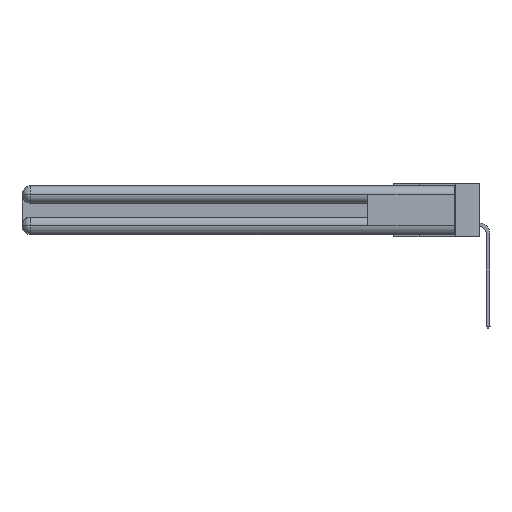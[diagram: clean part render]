
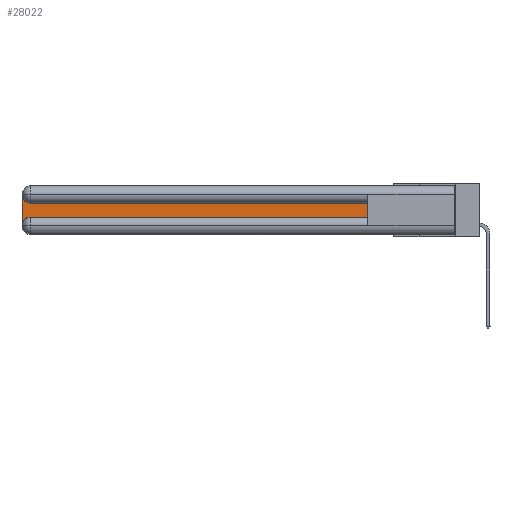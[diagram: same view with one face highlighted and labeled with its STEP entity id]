
A CAD part, left-side view. The second image highlights one B-rep face of the part: STEP entity #28022.
In plain terms, the highlighted planar face has unit normal (-1, 0, 0).
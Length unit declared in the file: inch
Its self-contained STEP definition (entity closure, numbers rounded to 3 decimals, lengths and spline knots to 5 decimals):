
#362 = CIRCLE ( 'NONE', #23428, 0.06 ) ;
#473 = ORIENTED_EDGE ( 'NONE', *, *, #30246, .T. ) ;
#719 = LINE ( 'NONE', #30095, #20214 ) ;
#2472 = ORIENTED_EDGE ( 'NONE', *, *, #22421, .T. ) ;
#3016 = CARTESIAN_POINT ( 'NONE',  ( 0.075, 2.94, -0.0625 ) ) ;
#3349 = VECTOR ( 'NONE', #31787, 39.37008 ) ;
#3365 = VERTEX_POINT ( 'NONE', #17235 ) ;
#3503 = PLANE ( 'NONE',  #10403 ) ;
#5571 = CIRCLE ( 'NONE', #5984, 0.06 ) ;
#5984 = AXIS2_PLACEMENT_3D ( 'NONE', #3016, #10112, #27837 ) ;
#6042 = VERTEX_POINT ( 'NONE', #25935 ) ;
#6546 = ORIENTED_EDGE ( 'NONE', *, *, #10411, .T. ) ;
#7723 = VERTEX_POINT ( 'NONE', #15657 ) ;
#8733 = DIRECTION ( 'NONE',  ( 0., 0., -1. ) ) ;
#9076 = ORIENTED_EDGE ( 'NONE', *, *, #14273, .T. ) ;
#9688 = CARTESIAN_POINT ( 'NONE',  ( 0.075, 2.94, -0.1225 ) ) ;
#10112 = DIRECTION ( 'NONE',  ( 1., 0., 0. ) ) ;
#10403 = AXIS2_PLACEMENT_3D ( 'NONE', #10964, #18632, #8733 ) ;
#10411 = EDGE_CURVE ( 'NONE', #28915, #12474, #24739, .T. ) ;
#10964 = CARTESIAN_POINT ( 'NONE',  ( 0.075, 3., -0.1225 ) ) ;
#11887 = DIRECTION ( 'NONE',  ( 0., 0., 1. ) ) ;
#12461 = DIRECTION ( 'NONE',  ( 0., 0., -1. ) ) ;
#12474 = VERTEX_POINT ( 'NONE', #30097 ) ;
#13506 = CARTESIAN_POINT ( 'NONE',  ( 0.075, 0.6, -0.2175 ) ) ;
#13574 = FACE_OUTER_BOUND ( 'NONE', #26102, .T. ) ;
#14273 = EDGE_CURVE ( 'NONE', #3365, #7723, #24403, .T. ) ;
#15581 = VECTOR ( 'NONE', #16238, 39.37008 ) ;
#15657 = CARTESIAN_POINT ( 'NONE',  ( 0.075, 3., -0.2775 ) ) ;
#15861 = CARTESIAN_POINT ( 'NONE',  ( 0.075, 0.6, -0.2175 ) ) ;
#16016 = VECTOR ( 'NONE', #11887, 39.37008 ) ;
#16238 = DIRECTION ( 'NONE',  ( 0., -1., 0. ) ) ;
#17235 = CARTESIAN_POINT ( 'NONE',  ( 0.075, 3., -0.0625 ) ) ;
#17311 = DIRECTION ( 'NONE',  ( 1., 0., 0. ) ) ;
#18632 = DIRECTION ( 'NONE',  ( 1., 0., 0. ) ) ;
#19292 = CARTESIAN_POINT ( 'NONE',  ( 0.075, 3., -0.2175 ) ) ;
#19768 = CARTESIAN_POINT ( 'NONE',  ( 0.075, 2.94, -0.2775 ) ) ;
#20214 = VECTOR ( 'NONE', #30424, 39.37008 ) ;
#21154 = LINE ( 'NONE', #13506, #15581 ) ;
#22421 = EDGE_CURVE ( 'NONE', #6042, #28915, #21154, .T. ) ;
#23117 = CARTESIAN_POINT ( 'NONE',  ( 0.075, 0.6, -0.2175 ) ) ;
#23428 = AXIS2_PLACEMENT_3D ( 'NONE', #19768, #17311, #12461 ) ;
#24403 = LINE ( 'NONE', #19292, #3349 ) ;
#24739 = LINE ( 'NONE', #23117, #16016 ) ;
#25345 = ORIENTED_EDGE ( 'NONE', *, *, #28622, .T. ) ;
#25935 = CARTESIAN_POINT ( 'NONE',  ( 0.075, 2.94, -0.2175 ) ) ;
#26102 = EDGE_LOOP ( 'NONE', ( #32805, #473, #9076, #25345, #2472, #6546 ) ) ;
#27837 = DIRECTION ( 'NONE',  ( 0., 0., -1. ) ) ;
#28022 = ADVANCED_FACE ( 'NONE', ( #13574 ), #3503, .F. ) ;
#28622 = EDGE_CURVE ( 'NONE', #7723, #6042, #362, .T. ) ;
#28915 = VERTEX_POINT ( 'NONE', #15861 ) ;
#29227 = EDGE_CURVE ( 'NONE', #12474, #30119, #719, .T. ) ;
#30095 = CARTESIAN_POINT ( 'NONE',  ( 0.075, 0.6, -0.1225 ) ) ;
#30097 = CARTESIAN_POINT ( 'NONE',  ( 0.075, 0.6, -0.1225 ) ) ;
#30119 = VERTEX_POINT ( 'NONE', #9688 ) ;
#30246 = EDGE_CURVE ( 'NONE', #30119, #3365, #5571, .T. ) ;
#30424 = DIRECTION ( 'NONE',  ( 0., 1., 0. ) ) ;
#31787 = DIRECTION ( 'NONE',  ( 0., 0., -1. ) ) ;
#32805 = ORIENTED_EDGE ( 'NONE', *, *, #29227, .T. ) ;
